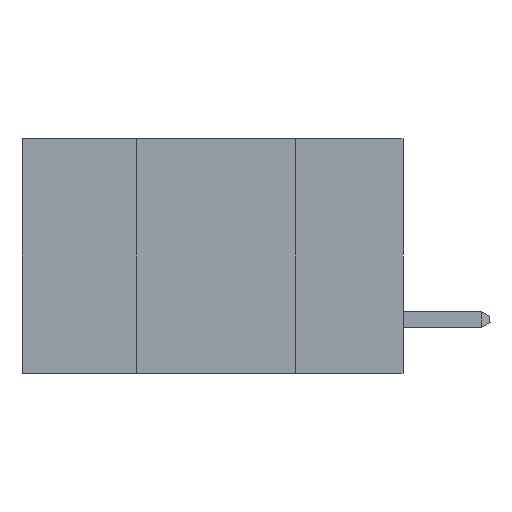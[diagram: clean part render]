
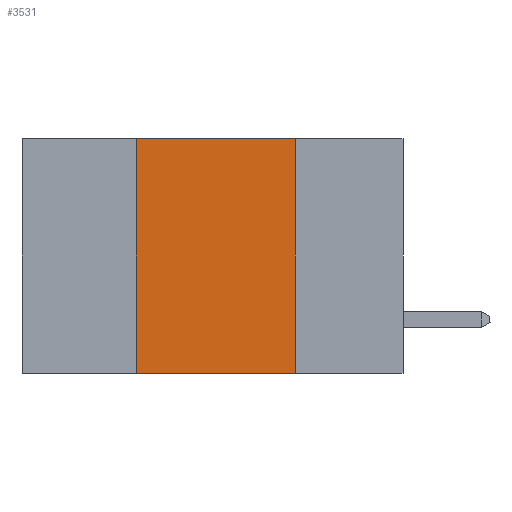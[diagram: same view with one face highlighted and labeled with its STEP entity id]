
A CAD part, left-side view. The second image highlights one B-rep face of the part: STEP entity #3531.
In plain terms, the highlighted planar face has unit normal (-1, 0, 0).
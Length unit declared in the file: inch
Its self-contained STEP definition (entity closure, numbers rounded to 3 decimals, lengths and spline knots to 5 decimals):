
#163 = VERTEX_POINT ( 'NONE', #18936 ) ;
#877 = LINE ( 'NONE', #5360, #6290 ) ;
#2532 = EDGE_CURVE ( 'NONE', #16794, #10757, #27171, .T. ) ;
#3531 = ADVANCED_FACE ( 'NONE', ( #24186 ), #30857, .F. ) ;
#4574 = ORIENTED_EDGE ( 'NONE', *, *, #32810, .T. ) ;
#5360 = CARTESIAN_POINT ( 'NONE',  ( 0., 0.6, -0.37 ) ) ;
#5633 = DIRECTION ( 'NONE',  ( 0., 0., 1. ) ) ;
#6290 = VECTOR ( 'NONE', #21457, 39.37008 ) ;
#7700 = VERTEX_POINT ( 'NONE', #37579 ) ;
#10757 = VERTEX_POINT ( 'NONE', #29526 ) ;
#11966 = CARTESIAN_POINT ( 'NONE',  ( 0., 0.6, 0. ) ) ;
#12097 = DIRECTION ( 'NONE',  ( 1., 0., 0. ) ) ;
#13530 = ORIENTED_EDGE ( 'NONE', *, *, #38019, .F. ) ;
#15198 = CARTESIAN_POINT ( 'NONE',  ( 0., 0.42, 0. ) ) ;
#15280 = CARTESIAN_POINT ( 'NONE',  ( 0., 0.6, 0. ) ) ;
#16010 = DIRECTION ( 'NONE',  ( 0., 0., -1. ) ) ;
#16794 = VERTEX_POINT ( 'NONE', #22742 ) ;
#18075 = LINE ( 'NONE', #15280, #23464 ) ;
#18625 = LINE ( 'NONE', #15198, #40887 ) ;
#18936 = CARTESIAN_POINT ( 'NONE',  ( 0., 0.42, 0. ) ) ;
#19870 = VECTOR ( 'NONE', #16010, 39.37008 ) ;
#21457 = DIRECTION ( 'NONE',  ( 0., -1., 0. ) ) ;
#22742 = CARTESIAN_POINT ( 'NONE',  ( 0., 0.17, 0. ) ) ;
#23464 = VECTOR ( 'NONE', #34478, 39.37008 ) ;
#24186 = FACE_OUTER_BOUND ( 'NONE', #26284, .T. ) ;
#25539 = ORIENTED_EDGE ( 'NONE', *, *, #38671, .F. ) ;
#26284 = EDGE_LOOP ( 'NONE', ( #33592, #25539, #13530, #4574 ) ) ;
#27171 = LINE ( 'NONE', #31983, #19870 ) ;
#28186 = AXIS2_PLACEMENT_3D ( 'NONE', #11966, #12097, #34070 ) ;
#29526 = CARTESIAN_POINT ( 'NONE',  ( 0., 0.17, -0.37 ) ) ;
#30857 = PLANE ( 'NONE',  #28186 ) ;
#31983 = CARTESIAN_POINT ( 'NONE',  ( 0., 0.17, 0. ) ) ;
#32810 = EDGE_CURVE ( 'NONE', #7700, #10757, #877, .T. ) ;
#33592 = ORIENTED_EDGE ( 'NONE', *, *, #2532, .F. ) ;
#34070 = DIRECTION ( 'NONE',  ( 0., 0., -1. ) ) ;
#34478 = DIRECTION ( 'NONE',  ( 0., -1., 0. ) ) ;
#37579 = CARTESIAN_POINT ( 'NONE',  ( 0., 0.42, -0.37 ) ) ;
#38019 = EDGE_CURVE ( 'NONE', #7700, #163, #18625, .T. ) ;
#38671 = EDGE_CURVE ( 'NONE', #163, #16794, #18075, .T. ) ;
#40887 = VECTOR ( 'NONE', #5633, 39.37008 ) ;
